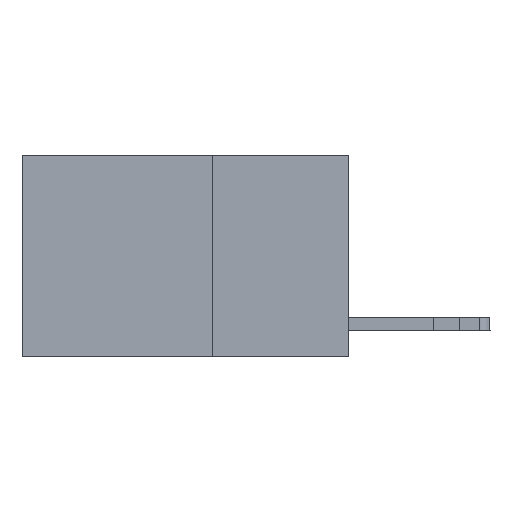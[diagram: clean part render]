
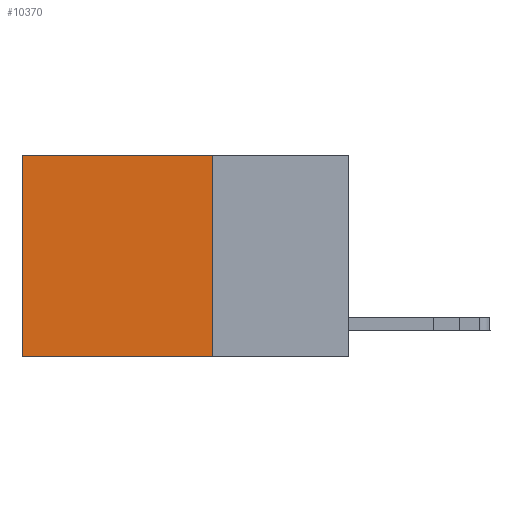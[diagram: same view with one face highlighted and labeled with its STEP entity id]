
A CAD part, left-side view. The second image highlights one B-rep face of the part: STEP entity #10370.
In plain terms, the highlighted planar face has unit normal (-1, 0, 0).
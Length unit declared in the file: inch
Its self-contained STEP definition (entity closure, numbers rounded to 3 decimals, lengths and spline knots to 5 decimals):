
#39 = FACE_OUTER_BOUND ( 'NONE', #3529, .T. ) ;
#173 = DIRECTION ( 'NONE',  ( 0., 0., -1. ) ) ;
#409 = VERTEX_POINT ( 'NONE', #15642 ) ;
#3529 = EDGE_LOOP ( 'NONE', ( #4359, #8586, #6876, #17278 ) ) ;
#4359 = ORIENTED_EDGE ( 'NONE', *, *, #11076, .T. ) ;
#4799 = EDGE_CURVE ( 'NONE', #15584, #12799, #6026, .T. ) ;
#5378 = EDGE_CURVE ( 'NONE', #409, #7072, #7711, .T. ) ;
#5476 = DIRECTION ( 'NONE',  ( 1., 0., 0. ) ) ;
#5892 = VECTOR ( 'NONE', #173, 39.37008 ) ;
#6026 = LINE ( 'NONE', #11493, #11533 ) ;
#6876 = ORIENTED_EDGE ( 'NONE', *, *, #10143, .F. ) ;
#7072 = VERTEX_POINT ( 'NONE', #13160 ) ;
#7517 = CARTESIAN_POINT ( 'NONE',  ( 0.2625, 0.6, 0. ) ) ;
#7711 = LINE ( 'NONE', #9149, #10969 ) ;
#8063 = DIRECTION ( 'NONE',  ( 0., 1., 0. ) ) ;
#8586 = ORIENTED_EDGE ( 'NONE', *, *, #4799, .F. ) ;
#8768 = LINE ( 'NONE', #7517, #11082 ) ;
#9149 = CARTESIAN_POINT ( 'NONE',  ( 0.2625, 0.25, 0. ) ) ;
#10143 = EDGE_CURVE ( 'NONE', #409, #15584, #13917, .T. ) ;
#10193 = DIRECTION ( 'NONE',  ( 0., 0., -1. ) ) ;
#10370 = ADVANCED_FACE ( 'NONE', ( #39 ), #15141, .F. ) ;
#10724 = CARTESIAN_POINT ( 'NONE',  ( 0.2625, 0.6, -0.37 ) ) ;
#10969 = VECTOR ( 'NONE', #8063, 39.37008 ) ;
#11076 = EDGE_CURVE ( 'NONE', #7072, #12799, #8768, .T. ) ;
#11082 = VECTOR ( 'NONE', #10193, 39.37008 ) ;
#11493 = CARTESIAN_POINT ( 'NONE',  ( 0.2625, 0.25, -0.37 ) ) ;
#11533 = VECTOR ( 'NONE', #16943, 39.37008 ) ;
#12692 = CARTESIAN_POINT ( 'NONE',  ( 0.2625, 0.25, 0. ) ) ;
#12799 = VERTEX_POINT ( 'NONE', #10724 ) ;
#13160 = CARTESIAN_POINT ( 'NONE',  ( 0.2625, 0.6, 0. ) ) ;
#13885 = DIRECTION ( 'NONE',  ( 0., 0., -1. ) ) ;
#13917 = LINE ( 'NONE', #12692, #5892 ) ;
#15141 = PLANE ( 'NONE',  #16493 ) ;
#15584 = VERTEX_POINT ( 'NONE', #16898 ) ;
#15642 = CARTESIAN_POINT ( 'NONE',  ( 0.2625, 0.25, 0. ) ) ;
#16493 = AXIS2_PLACEMENT_3D ( 'NONE', #16667, #5476, #13885 ) ;
#16667 = CARTESIAN_POINT ( 'NONE',  ( 0.2625, 0.25, 0. ) ) ;
#16898 = CARTESIAN_POINT ( 'NONE',  ( 0.2625, 0.25, -0.37 ) ) ;
#16943 = DIRECTION ( 'NONE',  ( 0., 1., 0. ) ) ;
#17278 = ORIENTED_EDGE ( 'NONE', *, *, #5378, .T. ) ;
